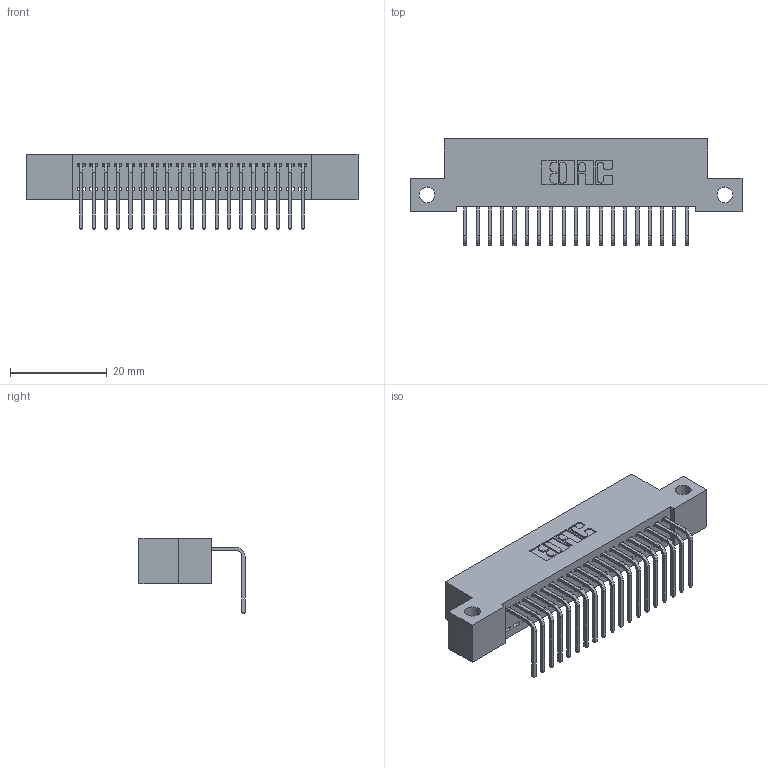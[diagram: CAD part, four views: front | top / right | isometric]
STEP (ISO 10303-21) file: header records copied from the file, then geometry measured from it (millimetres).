
FILE_DESCRIPTION (( 'STEP AP203' ), '1' );
FILE_NAME ('342-019-558-112.STEP', '2018-08-10T22:24:24', ( '' ), ( '' ), 'SwSTEP 2.0', 'SolidWorks 2016', '' );
FILE_SCHEMA (( 'CONFIG_CONTROL_DESIGN' ));
Length unit declared in the file: inch
Products named in the file (3): 342 Part_Side Mount; 345-292-001_558 Tail - 2; 342-019-558-112
Assembly tree (20 placements, depth 2):
  342-019-558-112
    342 Part_Side Mount
    345-292-001_558 Tail - 2  x19
Bounding box: 68.58 x 21.91 x 15.62 mm (x, y, z)
Volume: 5917.7 mm3; surface area: 8456.9 mm2
Topology: 20 solids, 20 shells, 1250 faces, 3757 edges, 2478 vertices
Faces by surface type: plane 902, cylinder 348
Entity records: 14545 total; most frequent: CARTESIAN_POINT 2519, ORIENTED_EDGE 2474, DIRECTION 2171, EDGE_CURVE 1237, VECTOR 1109, LINE 1109, VERTEX_POINT 822, AXIS2_PLACEMENT_3D 531
